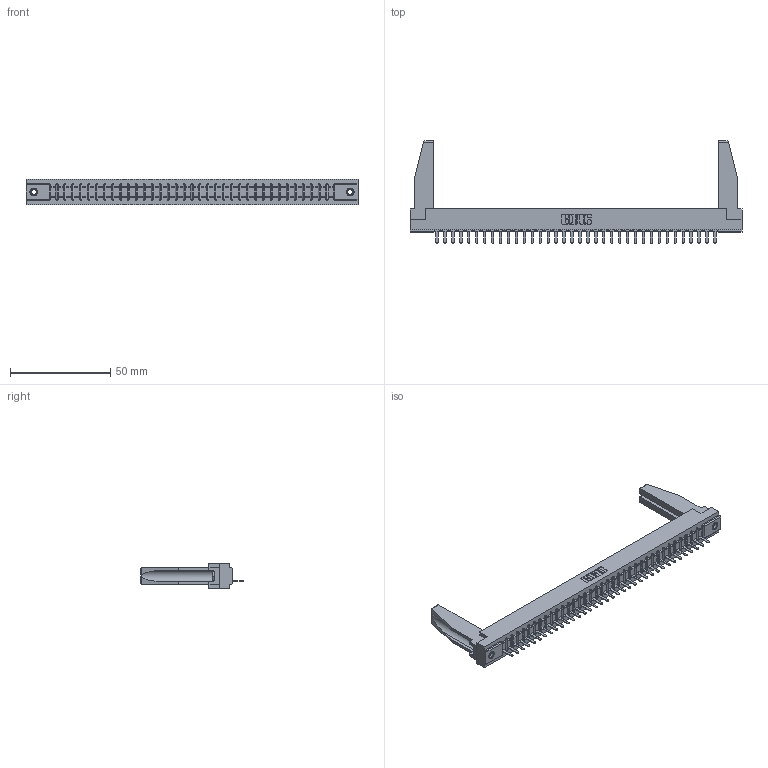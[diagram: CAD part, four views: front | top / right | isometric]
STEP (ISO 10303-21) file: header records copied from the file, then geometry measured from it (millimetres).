
FILE_DESCRIPTION (( 'STEP AP203' ), '1' );
FILE_NAME ('357-036-521-178.STEP', '2019-09-17T06:32:24', ( '' ), ( '' ), 'SwSTEP 2.0', 'SolidWorks 2016', '' );
FILE_SCHEMA (( 'CONFIG_CONTROL_DESIGN' ));
Length unit declared in the file: inch
Products named in the file (5): 345-250-001_345-250-001-102; 307-290-002_521; 307 Part_.156 Dia Mounting Holes; 307-220-078; 357-036-521-178
Assembly tree (41 placements, depth 2):
  357-036-521-178
    307 Part_.156 Dia Mounting Holes
    307-290-002_521  x36
    307-220-078  x2
    345-250-001_345-250-001-102  x2
Bounding box: 165.66 x 51.13 x 12.7 mm (x, y, z)
Volume: 21678.3 mm3; surface area: 25936.3 mm2
Topology: 41 solids, 41 shells, 2949 faces, 9005 edges, 5894 vertices
Faces by surface type: plane 1774, cylinder 1085, sphere 74, cone 12, torus 4
Entity records: 34759 total; most frequent: CARTESIAN_POINT 5862, ORIENTED_EDGE 5808, DIRECTION 5654, EDGE_CURVE 2904, VECTOR 2226, LINE 2226, VERTEX_POINT 1880, AXIS2_PLACEMENT_3D 1714
